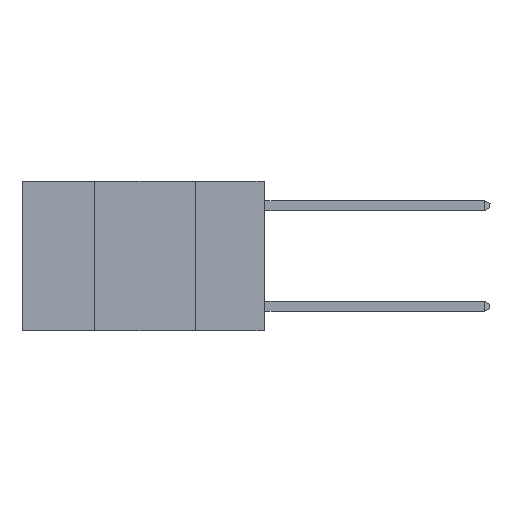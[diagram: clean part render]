
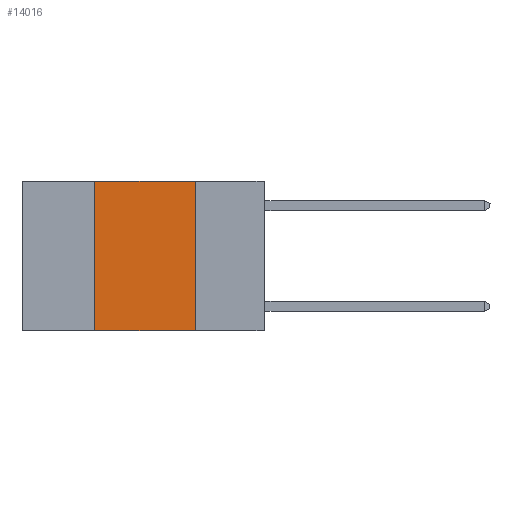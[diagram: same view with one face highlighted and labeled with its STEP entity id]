
A CAD part, left-side view. The second image highlights one B-rep face of the part: STEP entity #14016.
In plain terms, the highlighted planar face has unit normal (-1, 0, 0).
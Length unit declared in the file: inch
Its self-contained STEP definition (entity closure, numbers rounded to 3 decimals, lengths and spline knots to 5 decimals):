
#769 = VECTOR ( 'NONE', #12971, 39.37008 ) ;
#2020 = ORIENTED_EDGE ( 'NONE', *, *, #15018, .F. ) ;
#2248 = EDGE_CURVE ( 'NONE', #13440, #3553, #16464, .T. ) ;
#2249 = AXIS2_PLACEMENT_3D ( 'NONE', #5367, #6782, #2632 ) ;
#2632 = DIRECTION ( 'NONE',  ( 0., 0., -1. ) ) ;
#3553 = VERTEX_POINT ( 'NONE', #17501 ) ;
#4887 = EDGE_CURVE ( 'NONE', #16217, #11180, #16277, .T. ) ;
#5367 = CARTESIAN_POINT ( 'NONE',  ( 0., 0.6, 0. ) ) ;
#5407 = CARTESIAN_POINT ( 'NONE',  ( 0., 0.17, 0. ) ) ;
#5711 = LINE ( 'NONE', #7015, #769 ) ;
#6782 = DIRECTION ( 'NONE',  ( 1., 0., 0. ) ) ;
#7015 = CARTESIAN_POINT ( 'NONE',  ( 0., 0.42, 0. ) ) ;
#7190 = EDGE_LOOP ( 'NONE', ( #11914, #13669, #2020, #16907 ) ) ;
#8933 = VECTOR ( 'NONE', #9346, 39.37008 ) ;
#9346 = DIRECTION ( 'NONE',  ( 0., -1., 0. ) ) ;
#9747 = DIRECTION ( 'NONE',  ( 0., 0., -1. ) ) ;
#9932 = VECTOR ( 'NONE', #17778, 39.37008 ) ;
#10350 = EDGE_CURVE ( 'NONE', #3553, #11180, #13891, .T. ) ;
#11180 = VERTEX_POINT ( 'NONE', #11973 ) ;
#11606 = CARTESIAN_POINT ( 'NONE',  ( 0., 0.42, -0.37 ) ) ;
#11914 = ORIENTED_EDGE ( 'NONE', *, *, #10350, .F. ) ;
#11973 = CARTESIAN_POINT ( 'NONE',  ( 0., 0.17, -0.37 ) ) ;
#12971 = DIRECTION ( 'NONE',  ( 0., 0., 1. ) ) ;
#13440 = VERTEX_POINT ( 'NONE', #15213 ) ;
#13591 = CARTESIAN_POINT ( 'NONE',  ( 0., 0.6, -0.37 ) ) ;
#13669 = ORIENTED_EDGE ( 'NONE', *, *, #2248, .F. ) ;
#13891 = LINE ( 'NONE', #5407, #16753 ) ;
#13941 = FACE_OUTER_BOUND ( 'NONE', #7190, .T. ) ;
#14016 = ADVANCED_FACE ( 'NONE', ( #13941 ), #18414, .F. ) ;
#15018 = EDGE_CURVE ( 'NONE', #16217, #13440, #5711, .T. ) ;
#15213 = CARTESIAN_POINT ( 'NONE',  ( 0., 0.42, 0. ) ) ;
#16217 = VERTEX_POINT ( 'NONE', #11606 ) ;
#16277 = LINE ( 'NONE', #13591, #9932 ) ;
#16464 = LINE ( 'NONE', #16743, #8933 ) ;
#16743 = CARTESIAN_POINT ( 'NONE',  ( 0., 0.6, 0. ) ) ;
#16753 = VECTOR ( 'NONE', #9747, 39.37008 ) ;
#16907 = ORIENTED_EDGE ( 'NONE', *, *, #4887, .T. ) ;
#17501 = CARTESIAN_POINT ( 'NONE',  ( 0., 0.17, 0. ) ) ;
#17778 = DIRECTION ( 'NONE',  ( 0., -1., 0. ) ) ;
#18414 = PLANE ( 'NONE',  #2249 ) ;
